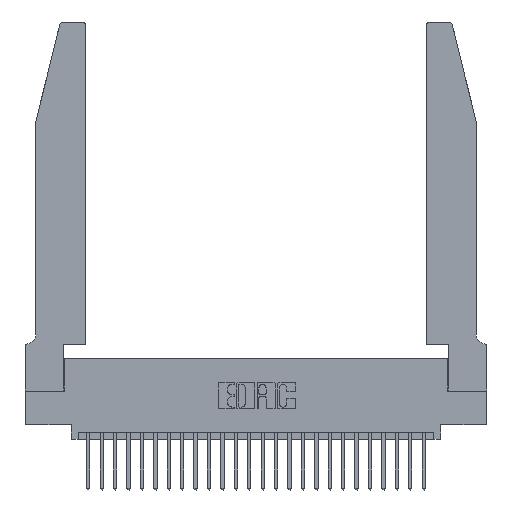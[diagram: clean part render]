
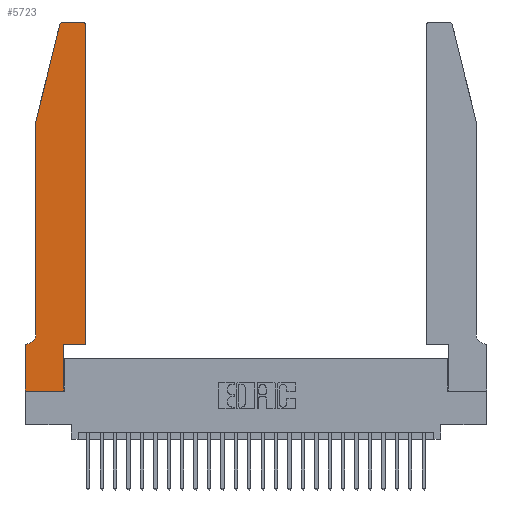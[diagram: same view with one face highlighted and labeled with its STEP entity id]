
A CAD part, top view. The second image highlights one B-rep face of the part: STEP entity #5723.
In plain terms, the highlighted planar face has unit normal (0, 0, 1).
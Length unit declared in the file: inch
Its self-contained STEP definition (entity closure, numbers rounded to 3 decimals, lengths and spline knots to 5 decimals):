
#389 = CARTESIAN_POINT ( 'NONE',  ( 0., 0.35, 0.37 ) ) ;
#735 = CARTESIAN_POINT ( 'NONE',  ( 0.4505, 0.35, 0.37 ) ) ;
#1241 = CARTESIAN_POINT ( 'NONE',  ( 0., 0., 0.37 ) ) ;
#1606 = LINE ( 'NONE', #18704, #13202 ) ;
#1632 = CARTESIAN_POINT ( 'NONE',  ( 0.4205, 2.72, 0.37 ) ) ;
#1750 = DIRECTION ( 'NONE',  ( 1., 0., 0. ) ) ;
#2200 = EDGE_CURVE ( 'NONE', #21121, #4723, #6340, .T. ) ;
#3213 = VERTEX_POINT ( 'NONE', #5982 ) ;
#3439 = EDGE_CURVE ( 'NONE', #6690, #19004, #23848, .T. ) ;
#3972 = ORIENTED_EDGE ( 'NONE', *, *, #22846, .T. ) ;
#4072 = PLANE ( 'NONE',  #6234 ) ;
#4309 = VERTEX_POINT ( 'NONE', #5363 ) ;
#4316 = VECTOR ( 'NONE', #8516, 39.37008 ) ;
#4596 = CARTESIAN_POINT ( 'NONE',  ( 0.284, 2.75, 0.37 ) ) ;
#4723 = VERTEX_POINT ( 'NONE', #19227 ) ;
#4743 = EDGE_CURVE ( 'NONE', #11043, #18288, #6836, .T. ) ;
#5026 = VERTEX_POINT ( 'NONE', #9869 ) ;
#5299 = ORIENTED_EDGE ( 'NONE', *, *, #14243, .T. ) ;
#5363 = CARTESIAN_POINT ( 'NONE',  ( 0., 0., 0.37 ) ) ;
#5421 = LINE ( 'NONE', #1241, #20995 ) ;
#5498 = CARTESIAN_POINT ( 'NONE',  ( 0.0755, 2., 0.37 ) ) ;
#5551 = EDGE_CURVE ( 'NONE', #4723, #9449, #23134, .T. ) ;
#5723 = ADVANCED_FACE ( 'NONE', ( #10187 ), #4072, .T. ) ;
#5917 = EDGE_CURVE ( 'NONE', #5026, #11043, #15504, .T. ) ;
#5982 = CARTESIAN_POINT ( 'NONE',  ( 0.0055, 0.35, 0.37 ) ) ;
#5992 = CARTESIAN_POINT ( 'NONE',  ( 0., 0.35, 0.37 ) ) ;
#5993 = VECTOR ( 'NONE', #20139, 39.37008 ) ;
#6234 = AXIS2_PLACEMENT_3D ( 'NONE', #5992, #10103, #1750 ) ;
#6340 = LINE ( 'NONE', #5498, #5993 ) ;
#6690 = VERTEX_POINT ( 'NONE', #20520 ) ;
#6836 = LINE ( 'NONE', #19316, #18801 ) ;
#6879 = CARTESIAN_POINT ( 'NONE',  ( 0.284, 2.72, 0.37 ) ) ;
#6966 = AXIS2_PLACEMENT_3D ( 'NONE', #6879, #6981, #23584 ) ;
#6981 = DIRECTION ( 'NONE',  ( 0., 0., 1. ) ) ;
#7092 = CARTESIAN_POINT ( 'NONE',  ( 0.4505, 0.35, 0.37 ) ) ;
#7278 = VECTOR ( 'NONE', #12221, 39.37008 ) ;
#7733 = ORIENTED_EDGE ( 'NONE', *, *, #5551, .T. ) ;
#7934 = EDGE_LOOP ( 'NONE', ( #13160, #18060, #14773, #7733, #3972, #17554, #13932, #21425, #5299, #11625, #24362, #11663 ) ) ;
#8516 = DIRECTION ( 'NONE',  ( -1., 0., 0. ) ) ;
#8811 = CIRCLE ( 'NONE', #24663, 0.07 ) ;
#8822 = VECTOR ( 'NONE', #15553, 39.37008 ) ;
#9449 = VERTEX_POINT ( 'NONE', #10488 ) ;
#9869 = CARTESIAN_POINT ( 'NONE',  ( 0.2865, 0.35, 0.37 ) ) ;
#9959 = LINE ( 'NONE', #12135, #7278 ) ;
#10033 = CARTESIAN_POINT ( 'NONE',  ( 0.0055, 0.42, 0.37 ) ) ;
#10103 = DIRECTION ( 'NONE',  ( 0., 0., 1. ) ) ;
#10187 = FACE_OUTER_BOUND ( 'NONE', #7934, .T. ) ;
#10488 = CARTESIAN_POINT ( 'NONE',  ( 0.0755, 0.42, 0.37 ) ) ;
#10983 = DIRECTION ( 'NONE',  ( 0., 1., 0. ) ) ;
#11043 = VERTEX_POINT ( 'NONE', #735 ) ;
#11566 = DIRECTION ( 'NONE',  ( 0., 1., 0. ) ) ;
#11625 = ORIENTED_EDGE ( 'NONE', *, *, #5917, .T. ) ;
#11663 = ORIENTED_EDGE ( 'NONE', *, *, #27237, .T. ) ;
#11976 = VECTOR ( 'NONE', #11566, 39.37008 ) ;
#12133 = VERTEX_POINT ( 'NONE', #389 ) ;
#12135 = CARTESIAN_POINT ( 'NONE',  ( 0.0755, 0.35, 0.37 ) ) ;
#12221 = DIRECTION ( 'NONE',  ( -1., 0., 0. ) ) ;
#12818 = AXIS2_PLACEMENT_3D ( 'NONE', #1632, #16629, #20731 ) ;
#13160 = ORIENTED_EDGE ( 'NONE', *, *, #3439, .T. ) ;
#13174 = VECTOR ( 'NONE', #19833, 39.37008 ) ;
#13202 = VECTOR ( 'NONE', #14368, 39.37008 ) ;
#13932 = ORIENTED_EDGE ( 'NONE', *, *, #19254, .T. ) ;
#14243 = EDGE_CURVE ( 'NONE', #21175, #5026, #17590, .T. ) ;
#14368 = DIRECTION ( 'NONE',  ( 1., 0., 0. ) ) ;
#14374 = CARTESIAN_POINT ( 'NONE',  ( 0.4505, 2.72, 0.37 ) ) ;
#14773 = ORIENTED_EDGE ( 'NONE', *, *, #2200, .T. ) ;
#15504 = LINE ( 'NONE', #7092, #8822 ) ;
#15553 = DIRECTION ( 'NONE',  ( 1., 0., 0. ) ) ;
#15599 = EDGE_CURVE ( 'NONE', #4309, #21175, #1606, .T. ) ;
#16629 = DIRECTION ( 'NONE',  ( 0., 0., 1. ) ) ;
#17554 = ORIENTED_EDGE ( 'NONE', *, *, #20809, .T. ) ;
#17590 = LINE ( 'NONE', #18039, #11976 ) ;
#18039 = CARTESIAN_POINT ( 'NONE',  ( 0.2865, 0.35, 0.37 ) ) ;
#18060 = ORIENTED_EDGE ( 'NONE', *, *, #19020, .T. ) ;
#18288 = VERTEX_POINT ( 'NONE', #14374 ) ;
#18704 = CARTESIAN_POINT ( 'NONE',  ( 0., 0., 0.37 ) ) ;
#18801 = VECTOR ( 'NONE', #10983, 39.37008 ) ;
#19004 = VERTEX_POINT ( 'NONE', #4596 ) ;
#19020 = EDGE_CURVE ( 'NONE', #19004, #21121, #21355, .T. ) ;
#19227 = CARTESIAN_POINT ( 'NONE',  ( 0.0755, 2., 0.37 ) ) ;
#19254 = EDGE_CURVE ( 'NONE', #12133, #4309, #5421, .T. ) ;
#19316 = CARTESIAN_POINT ( 'NONE',  ( 0.4505, 0.35, 0.37 ) ) ;
#19418 = CARTESIAN_POINT ( 'NONE',  ( 0.25487, 2.72718, 0.37 ) ) ;
#19833 = DIRECTION ( 'NONE',  ( 0., -1., 0. ) ) ;
#20139 = DIRECTION ( 'NONE',  ( -0.239, -0.971, 0. ) ) ;
#20520 = CARTESIAN_POINT ( 'NONE',  ( 0.4205, 2.75, 0.37 ) ) ;
#20731 = DIRECTION ( 'NONE',  ( 1., 0., 0. ) ) ;
#20809 = EDGE_CURVE ( 'NONE', #3213, #12133, #9959, .T. ) ;
#20995 = VECTOR ( 'NONE', #26931, 39.37008 ) ;
#21087 = DIRECTION ( 'NONE',  ( -1., 0., 0. ) ) ;
#21121 = VERTEX_POINT ( 'NONE', #19418 ) ;
#21175 = VERTEX_POINT ( 'NONE', #25805 ) ;
#21246 = CARTESIAN_POINT ( 'NONE',  ( 0.2605, 2.75, 0.37 ) ) ;
#21355 = CIRCLE ( 'NONE', #6966, 0.03 ) ;
#21425 = ORIENTED_EDGE ( 'NONE', *, *, #15599, .T. ) ;
#22846 = EDGE_CURVE ( 'NONE', #9449, #3213, #8811, .T. ) ;
#23134 = LINE ( 'NONE', #26142, #13174 ) ;
#23584 = DIRECTION ( 'NONE',  ( 1., 0., 0. ) ) ;
#23848 = LINE ( 'NONE', #21246, #4316 ) ;
#24352 = CIRCLE ( 'NONE', #12818, 0.03 ) ;
#24362 = ORIENTED_EDGE ( 'NONE', *, *, #4743, .T. ) ;
#24663 = AXIS2_PLACEMENT_3D ( 'NONE', #10033, #25901, #21087 ) ;
#25805 = CARTESIAN_POINT ( 'NONE',  ( 0.2865, 0., 0.37 ) ) ;
#25901 = DIRECTION ( 'NONE',  ( 0., 0., -1. ) ) ;
#26142 = CARTESIAN_POINT ( 'NONE',  ( 0.0755, 2., 0.37 ) ) ;
#26931 = DIRECTION ( 'NONE',  ( 0., -1., 0. ) ) ;
#27237 = EDGE_CURVE ( 'NONE', #18288, #6690, #24352, .T. ) ;
